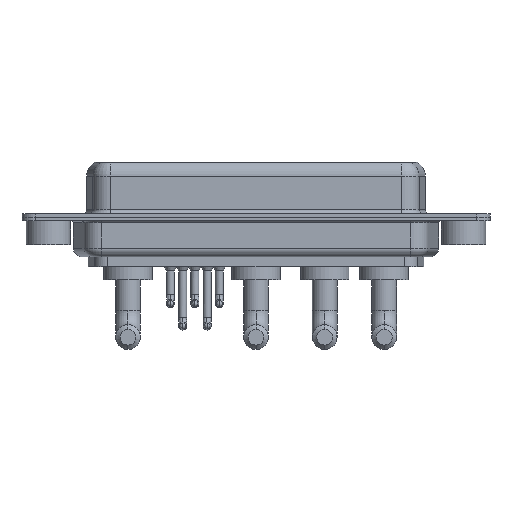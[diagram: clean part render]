
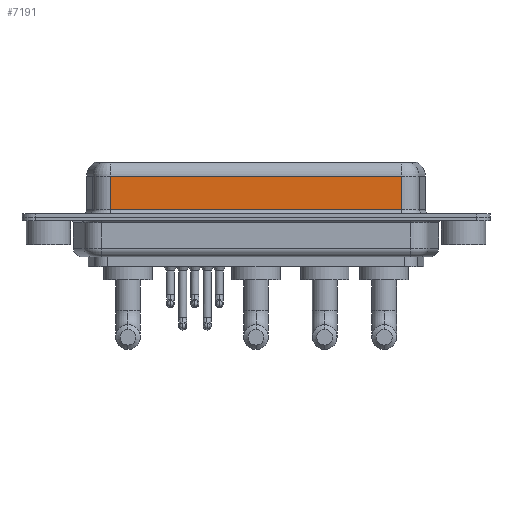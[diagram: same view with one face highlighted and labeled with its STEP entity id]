
A CAD part, front view. The second image highlights one B-rep face of the part: STEP entity #7191.
In plain terms, the highlighted planar face has unit normal (0, -1, 0).
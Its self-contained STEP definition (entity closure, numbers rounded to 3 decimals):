
#126 = DIRECTION ( 'NONE',  ( 0., 0., -1. ) ) ;
#209 = LINE ( 'NONE', #5408, #979 ) ;
#426 = ORIENTED_EDGE ( 'NONE', *, *, #13208, .T. ) ;
#712 = CARTESIAN_POINT ( 'NONE',  ( 40.037, -3.95, 4.65 ) ) ;
#887 = CARTESIAN_POINT ( 'NONE',  ( 40.037, -3.95, 0.9 ) ) ;
#933 = DIRECTION ( 'NONE',  ( 1., 0., 0. ) ) ;
#979 = VECTOR ( 'NONE', #126, 1000. ) ;
#1646 = CARTESIAN_POINT ( 'NONE',  ( 7.013, -3.95, 0.9 ) ) ;
#2610 = DIRECTION ( 'NONE',  ( 0., 0., 1. ) ) ;
#2718 = EDGE_CURVE ( 'NONE', #14213, #6763, #8792, .T. ) ;
#3449 = ORIENTED_EDGE ( 'NONE', *, *, #7806, .T. ) ;
#3843 = VECTOR ( 'NONE', #14406, 1000. ) ;
#5175 = LINE ( 'NONE', #6421, #14855 ) ;
#5408 = CARTESIAN_POINT ( 'NONE',  ( 7.013, -3.95, 6.4 ) ) ;
#5477 = ORIENTED_EDGE ( 'NONE', *, *, #2718, .T. ) ;
#6291 = LINE ( 'NONE', #16944, #3843 ) ;
#6421 = CARTESIAN_POINT ( 'NONE',  ( 40.037, -3.95, 0.9 ) ) ;
#6692 = EDGE_LOOP ( 'NONE', ( #8672, #5477, #3449, #426 ) ) ;
#6763 = VERTEX_POINT ( 'NONE', #12092 ) ;
#7191 = ADVANCED_FACE ( 'NONE', ( #7826 ), #9289, .F. ) ;
#7806 = EDGE_CURVE ( 'NONE', #6763, #14918, #209, .T. ) ;
#7826 = FACE_OUTER_BOUND ( 'NONE', #6692, .T. ) ;
#8664 = CARTESIAN_POINT ( 'NONE',  ( 40.037, -3.95, 4.65 ) ) ;
#8672 = ORIENTED_EDGE ( 'NONE', *, *, #9423, .F. ) ;
#8792 = LINE ( 'NONE', #712, #17157 ) ;
#9289 = PLANE ( 'NONE',  #13037 ) ;
#9423 = EDGE_CURVE ( 'NONE', #14213, #12684, #6291, .T. ) ;
#12092 = CARTESIAN_POINT ( 'NONE',  ( 7.013, -3.95, 4.65 ) ) ;
#12684 = VERTEX_POINT ( 'NONE', #887 ) ;
#13037 = AXIS2_PLACEMENT_3D ( 'NONE', #13142, #14617, #2610 ) ;
#13142 = CARTESIAN_POINT ( 'NONE',  ( 40.037, -3.95, 6.4 ) ) ;
#13208 = EDGE_CURVE ( 'NONE', #14918, #12684, #5175, .T. ) ;
#14213 = VERTEX_POINT ( 'NONE', #8664 ) ;
#14406 = DIRECTION ( 'NONE',  ( 0., 0., -1. ) ) ;
#14617 = DIRECTION ( 'NONE',  ( 0., 1., 0. ) ) ;
#14855 = VECTOR ( 'NONE', #933, 1000. ) ;
#14918 = VERTEX_POINT ( 'NONE', #1646 ) ;
#16732 = DIRECTION ( 'NONE',  ( -1., 0., 0. ) ) ;
#16944 = CARTESIAN_POINT ( 'NONE',  ( 40.037, -3.95, 6.4 ) ) ;
#17157 = VECTOR ( 'NONE', #16732, 1000. ) ;
